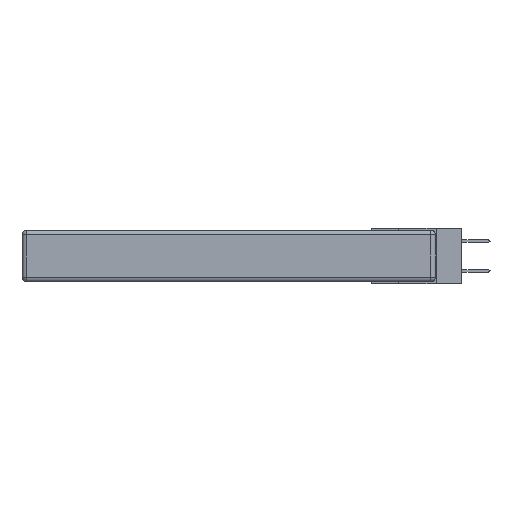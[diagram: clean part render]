
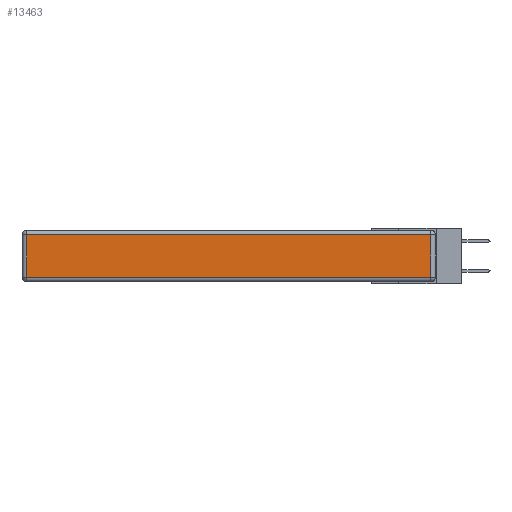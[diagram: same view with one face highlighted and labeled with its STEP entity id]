
A CAD part, left-side view. The second image highlights one B-rep face of the part: STEP entity #13463.
In plain terms, the highlighted planar face has unit normal (-1, 0, 0).
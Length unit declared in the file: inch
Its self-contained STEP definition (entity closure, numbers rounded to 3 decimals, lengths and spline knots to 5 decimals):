
#1311 = FACE_OUTER_BOUND ( 'NONE', #1439, .T. ) ;
#1439 = EDGE_LOOP ( 'NONE', ( #12637, #8306, #14573, #10311 ) ) ;
#1739 = VERTEX_POINT ( 'NONE', #8979 ) ;
#2688 = LINE ( 'NONE', #10555, #12409 ) ;
#2836 = CARTESIAN_POINT ( 'NONE',  ( 0., 2.75, -0.03 ) ) ;
#2992 = CARTESIAN_POINT ( 'NONE',  ( 0., 2.72, -0.03 ) ) ;
#4007 = VERTEX_POINT ( 'NONE', #2992 ) ;
#4653 = LINE ( 'NONE', #14825, #15639 ) ;
#5161 = DIRECTION ( 'NONE',  ( 0., 0., -1. ) ) ;
#5279 = PLANE ( 'NONE',  #12700 ) ;
#5390 = DIRECTION ( 'NONE',  ( 0., -1., 0. ) ) ;
#5762 = EDGE_CURVE ( 'NONE', #1739, #4007, #10630, .T. ) ;
#7292 = VERTEX_POINT ( 'NONE', #12626 ) ;
#7454 = VECTOR ( 'NONE', #8224, 39.37008 ) ;
#7841 = VERTEX_POINT ( 'NONE', #13171 ) ;
#8103 = EDGE_CURVE ( 'NONE', #7841, #1739, #14794, .T. ) ;
#8224 = DIRECTION ( 'NONE',  ( 0., 1., 0. ) ) ;
#8306 = ORIENTED_EDGE ( 'NONE', *, *, #8103, .T. ) ;
#8728 = EDGE_CURVE ( 'NONE', #7292, #7841, #4653, .T. ) ;
#8979 = CARTESIAN_POINT ( 'NONE',  ( 0., 0.03, -0.03 ) ) ;
#9370 = DIRECTION ( 'NONE',  ( -1., 0., 0. ) ) ;
#10311 = ORIENTED_EDGE ( 'NONE', *, *, #16234, .T. ) ;
#10555 = CARTESIAN_POINT ( 'NONE',  ( 0., 2.72, -0.343 ) ) ;
#10626 = CARTESIAN_POINT ( 'NONE',  ( 0., 0.03, -0.343 ) ) ;
#10630 = LINE ( 'NONE', #2836, #7454 ) ;
#12409 = VECTOR ( 'NONE', #5161, 39.37008 ) ;
#12626 = CARTESIAN_POINT ( 'NONE',  ( 0., 2.72, -0.313 ) ) ;
#12637 = ORIENTED_EDGE ( 'NONE', *, *, #8728, .T. ) ;
#12700 = AXIS2_PLACEMENT_3D ( 'NONE', #17461, #9370, #14552 ) ;
#13171 = CARTESIAN_POINT ( 'NONE',  ( 0., 0.03, -0.313 ) ) ;
#13347 = DIRECTION ( 'NONE',  ( 0., 0., 1. ) ) ;
#13463 = ADVANCED_FACE ( 'NONE', ( #1311 ), #5279, .T. ) ;
#14552 = DIRECTION ( 'NONE',  ( 0., 0., 1. ) ) ;
#14573 = ORIENTED_EDGE ( 'NONE', *, *, #5762, .T. ) ;
#14794 = LINE ( 'NONE', #10626, #17151 ) ;
#14825 = CARTESIAN_POINT ( 'NONE',  ( 0., 0., -0.313 ) ) ;
#15639 = VECTOR ( 'NONE', #5390, 39.37008 ) ;
#16234 = EDGE_CURVE ( 'NONE', #4007, #7292, #2688, .T. ) ;
#17151 = VECTOR ( 'NONE', #13347, 39.37008 ) ;
#17461 = CARTESIAN_POINT ( 'NONE',  ( 0., 0., -0.343 ) ) ;
